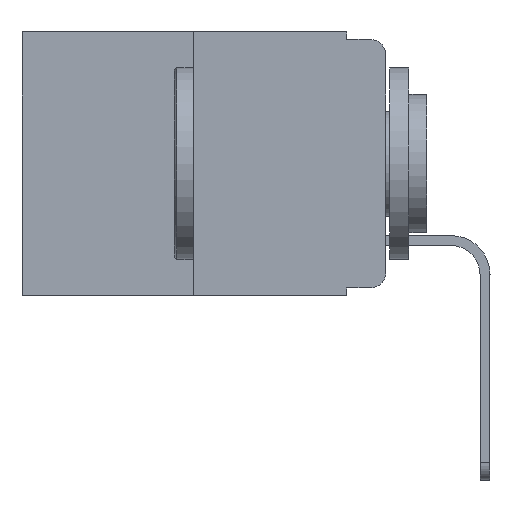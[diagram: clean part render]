
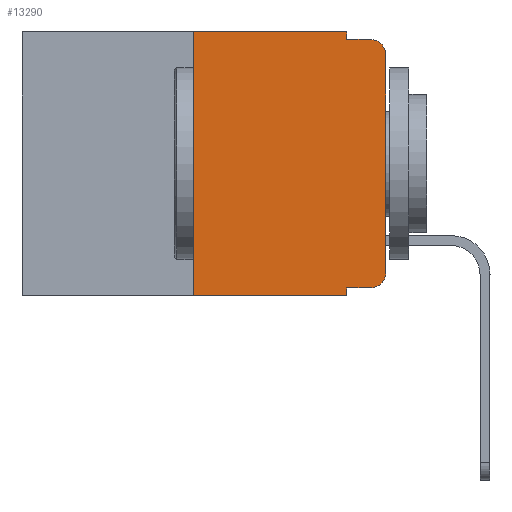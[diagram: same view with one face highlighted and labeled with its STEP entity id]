
A CAD part, left-side view. The second image highlights one B-rep face of the part: STEP entity #13290.
In plain terms, the highlighted planar face has unit normal (-1, 0, 0).
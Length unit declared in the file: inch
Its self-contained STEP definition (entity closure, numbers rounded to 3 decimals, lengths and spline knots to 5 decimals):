
#162 = VERTEX_POINT ( 'NONE', #21875 ) ;
#576 = VERTEX_POINT ( 'NONE', #5259 ) ;
#614 = ORIENTED_EDGE ( 'NONE', *, *, #13038, .T. ) ;
#883 = LINE ( 'NONE', #18183, #14542 ) ;
#914 = CARTESIAN_POINT ( 'NONE',  ( 0., 0., -0.03 ) ) ;
#1560 = EDGE_CURVE ( 'NONE', #576, #3646, #10820, .T. ) ;
#2753 = AXIS2_PLACEMENT_3D ( 'NONE', #20590, #8292, #4872 ) ;
#3249 = ORIENTED_EDGE ( 'NONE', *, *, #9157, .T. ) ;
#3492 = AXIS2_PLACEMENT_3D ( 'NONE', #15303, #6442, #18937 ) ;
#3543 = DIRECTION ( 'NONE',  ( 0., 0., -1. ) ) ;
#3616 = CARTESIAN_POINT ( 'NONE',  ( 0., 0.051, 0. ) ) ;
#3646 = VERTEX_POINT ( 'NONE', #20661 ) ;
#3744 = VECTOR ( 'NONE', #3543, 39.37008 ) ;
#4034 = ORIENTED_EDGE ( 'NONE', *, *, #15380, .F. ) ;
#4035 = ORIENTED_EDGE ( 'NONE', *, *, #16538, .T. ) ;
#4872 = DIRECTION ( 'NONE',  ( 0., 0., -1. ) ) ;
#5051 = ORIENTED_EDGE ( 'NONE', *, *, #9915, .F. ) ;
#5118 = VERTEX_POINT ( 'NONE', #10773 ) ;
#5161 = DIRECTION ( 'NONE',  ( 0., -1., 0. ) ) ;
#5259 = CARTESIAN_POINT ( 'NONE',  ( 0., 0.051, 0. ) ) ;
#5667 = CARTESIAN_POINT ( 'NONE',  ( 0., 0.25, 0. ) ) ;
#5805 = LINE ( 'NONE', #11353, #22631 ) ;
#6042 = DIRECTION ( 'NONE',  ( 0., 0., 1. ) ) ;
#6064 = FACE_OUTER_BOUND ( 'NONE', #14055, .T. ) ;
#6096 = VECTOR ( 'NONE', #16371, 39.37008 ) ;
#6434 = ORIENTED_EDGE ( 'NONE', *, *, #20039, .T. ) ;
#6442 = DIRECTION ( 'NONE',  ( -1., 0., 0. ) ) ;
#6568 = CIRCLE ( 'NONE', #2753, 0.02 ) ;
#6654 = EDGE_CURVE ( 'NONE', #21836, #9795, #7194, .T. ) ;
#6689 = DIRECTION ( 'NONE',  ( 0., -1., 0. ) ) ;
#6762 = CARTESIAN_POINT ( 'NONE',  ( 0., 0.473, 0. ) ) ;
#6873 = CARTESIAN_POINT ( 'NONE',  ( 0., 0.051, -0.01 ) ) ;
#7194 = LINE ( 'NONE', #5667, #15551 ) ;
#7313 = VECTOR ( 'NONE', #7476, 39.37008 ) ;
#7476 = DIRECTION ( 'NONE',  ( 0., -1., 0. ) ) ;
#7653 = ORIENTED_EDGE ( 'NONE', *, *, #1560, .F. ) ;
#7887 = VECTOR ( 'NONE', #5161, 39.37008 ) ;
#7906 = VERTEX_POINT ( 'NONE', #914 ) ;
#8245 = PLANE ( 'NONE',  #10461 ) ;
#8292 = DIRECTION ( 'NONE',  ( -1., 0., 0. ) ) ;
#8316 = CARTESIAN_POINT ( 'NONE',  ( 0., 0.473, 0. ) ) ;
#8550 = DIRECTION ( 'NONE',  ( 1., 0., 0. ) ) ;
#8665 = LINE ( 'NONE', #8316, #17593 ) ;
#9157 = EDGE_CURVE ( 'NONE', #21709, #10081, #6568, .T. ) ;
#9795 = VERTEX_POINT ( 'NONE', #10521 ) ;
#9915 = EDGE_CURVE ( 'NONE', #3646, #13996, #12910, .T. ) ;
#10081 = VERTEX_POINT ( 'NONE', #18463 ) ;
#10248 = CARTESIAN_POINT ( 'NONE',  ( 0., 0.02, -0.01 ) ) ;
#10461 = AXIS2_PLACEMENT_3D ( 'NONE', #6762, #8550, #21011 ) ;
#10521 = CARTESIAN_POINT ( 'NONE',  ( 0., 0.25, 0. ) ) ;
#10749 = ORIENTED_EDGE ( 'NONE', *, *, #6654, .F. ) ;
#10773 = CARTESIAN_POINT ( 'NONE',  ( 0., 0.051, -0.333 ) ) ;
#10820 = LINE ( 'NONE', #18105, #6096 ) ;
#10995 = CARTESIAN_POINT ( 'NONE',  ( 0., 0.051, -0.333 ) ) ;
#11353 = CARTESIAN_POINT ( 'NONE',  ( 0., 0.473, -0.343 ) ) ;
#11428 = DIRECTION ( 'NONE',  ( 0., 0., 1. ) ) ;
#12619 = ORIENTED_EDGE ( 'NONE', *, *, #19942, .T. ) ;
#12910 = LINE ( 'NONE', #6873, #7887 ) ;
#13038 = EDGE_CURVE ( 'NONE', #21836, #162, #5805, .T. ) ;
#13213 = LINE ( 'NONE', #3616, #3744 ) ;
#13290 = ADVANCED_FACE ( 'NONE', ( #6064 ), #8245, .F. ) ;
#13421 = LINE ( 'NONE', #10995, #7313 ) ;
#13996 = VERTEX_POINT ( 'NONE', #10248 ) ;
#14055 = EDGE_LOOP ( 'NONE', ( #6434, #4035, #5051, #7653, #17590, #10749, #614, #4034, #12619, #3249 ) ) ;
#14542 = VECTOR ( 'NONE', #11428, 39.37008 ) ;
#14953 = DIRECTION ( 'NONE',  ( 0., -1., 0. ) ) ;
#15303 = CARTESIAN_POINT ( 'NONE',  ( 0., 0.02, -0.03 ) ) ;
#15380 = EDGE_CURVE ( 'NONE', #5118, #162, #13213, .T. ) ;
#15417 = CARTESIAN_POINT ( 'NONE',  ( 0., 0.25, -0.343 ) ) ;
#15551 = VECTOR ( 'NONE', #6042, 39.37008 ) ;
#16371 = DIRECTION ( 'NONE',  ( 0., 0., -1. ) ) ;
#16538 = EDGE_CURVE ( 'NONE', #7906, #13996, #22760, .T. ) ;
#17590 = ORIENTED_EDGE ( 'NONE', *, *, #21817, .F. ) ;
#17593 = VECTOR ( 'NONE', #6689, 39.37008 ) ;
#18105 = CARTESIAN_POINT ( 'NONE',  ( 0., 0.051, 0. ) ) ;
#18183 = CARTESIAN_POINT ( 'NONE',  ( 0., 0., 0. ) ) ;
#18463 = CARTESIAN_POINT ( 'NONE',  ( 0., 0., -0.313 ) ) ;
#18937 = DIRECTION ( 'NONE',  ( 0., 0., -1. ) ) ;
#19001 = CARTESIAN_POINT ( 'NONE',  ( 0., 0.02, -0.333 ) ) ;
#19942 = EDGE_CURVE ( 'NONE', #5118, #21709, #13421, .T. ) ;
#20039 = EDGE_CURVE ( 'NONE', #10081, #7906, #883, .T. ) ;
#20590 = CARTESIAN_POINT ( 'NONE',  ( 0., 0.02, -0.313 ) ) ;
#20661 = CARTESIAN_POINT ( 'NONE',  ( 0., 0.051, -0.01 ) ) ;
#21011 = DIRECTION ( 'NONE',  ( 0., 0., -1. ) ) ;
#21709 = VERTEX_POINT ( 'NONE', #19001 ) ;
#21817 = EDGE_CURVE ( 'NONE', #9795, #576, #8665, .T. ) ;
#21836 = VERTEX_POINT ( 'NONE', #15417 ) ;
#21875 = CARTESIAN_POINT ( 'NONE',  ( 0., 0.051, -0.343 ) ) ;
#22631 = VECTOR ( 'NONE', #14953, 39.37008 ) ;
#22760 = CIRCLE ( 'NONE', #3492, 0.02 ) ;
